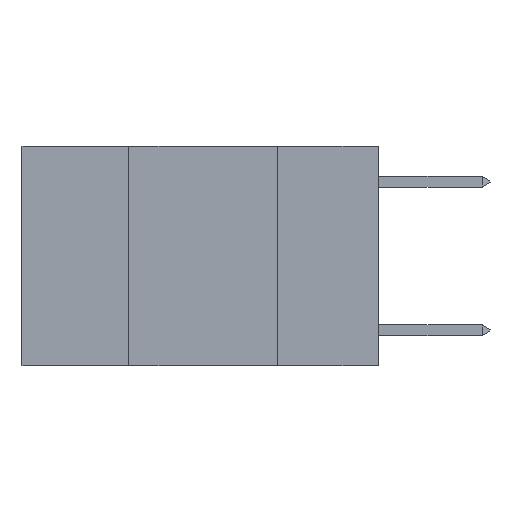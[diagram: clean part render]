
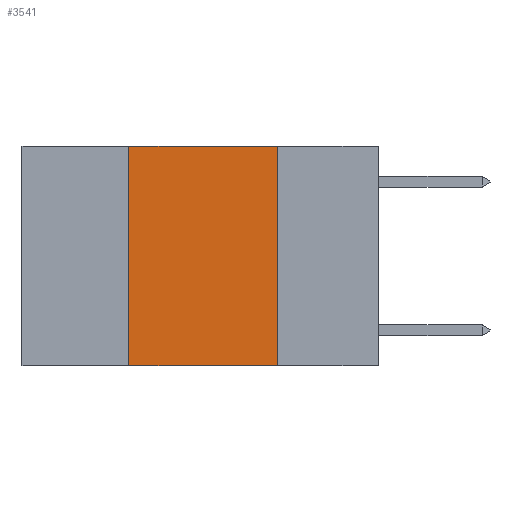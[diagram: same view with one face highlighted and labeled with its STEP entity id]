
A CAD part, left-side view. The second image highlights one B-rep face of the part: STEP entity #3541.
In plain terms, the highlighted planar face has unit normal (-1, 0, 0).
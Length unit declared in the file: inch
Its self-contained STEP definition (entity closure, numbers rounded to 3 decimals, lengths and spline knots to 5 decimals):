
#386 = ORIENTED_EDGE ( 'NONE', *, *, #5885, .F. ) ;
#1337 = VERTEX_POINT ( 'NONE', #8611 ) ;
#1564 = VECTOR ( 'NONE', #6463, 39.37008 ) ;
#2106 = VECTOR ( 'NONE', #2562, 39.37008 ) ;
#2552 = CARTESIAN_POINT ( 'NONE',  ( 0., 0.6, -0.37 ) ) ;
#2562 = DIRECTION ( 'NONE',  ( 0., -1., 0. ) ) ;
#2815 = ORIENTED_EDGE ( 'NONE', *, *, #5584, .F. ) ;
#3263 = LINE ( 'NONE', #6498, #1564 ) ;
#3357 = ORIENTED_EDGE ( 'NONE', *, *, #6048, .T. ) ;
#3540 = VERTEX_POINT ( 'NONE', #3819 ) ;
#3541 = ADVANCED_FACE ( 'NONE', ( #12477 ), #3782, .F. ) ;
#3711 = DIRECTION ( 'NONE',  ( 0., 0., -1. ) ) ;
#3741 = DIRECTION ( 'NONE',  ( 1., 0., 0. ) ) ;
#3755 = CARTESIAN_POINT ( 'NONE',  ( 0., 0.6, 0. ) ) ;
#3782 = PLANE ( 'NONE',  #4789 ) ;
#3798 = CARTESIAN_POINT ( 'NONE',  ( 0., 0.17, 0. ) ) ;
#3811 = DIRECTION ( 'NONE',  ( 0., 0., 1. ) ) ;
#3819 = CARTESIAN_POINT ( 'NONE',  ( 0., 0.42, -0.37 ) ) ;
#3984 = CARTESIAN_POINT ( 'NONE',  ( 0., 0.42, 0. ) ) ;
#4105 = LINE ( 'NONE', #2552, #2106 ) ;
#4789 = AXIS2_PLACEMENT_3D ( 'NONE', #3755, #3741, #3711 ) ;
#5584 = EDGE_CURVE ( 'NONE', #9605, #1337, #3263, .T. ) ;
#5885 = EDGE_CURVE ( 'NONE', #3540, #11742, #9350, .T. ) ;
#6048 = EDGE_CURVE ( 'NONE', #3540, #1337, #4105, .T. ) ;
#6463 = DIRECTION ( 'NONE',  ( 0., 0., -1. ) ) ;
#6498 = CARTESIAN_POINT ( 'NONE',  ( 0., 0.17, 0. ) ) ;
#7395 = VECTOR ( 'NONE', #8224, 39.37008 ) ;
#7865 = CARTESIAN_POINT ( 'NONE',  ( 0., 0.42, 0. ) ) ;
#8224 = DIRECTION ( 'NONE',  ( 0., -1., 0. ) ) ;
#8611 = CARTESIAN_POINT ( 'NONE',  ( 0., 0.17, -0.37 ) ) ;
#9176 = VECTOR ( 'NONE', #3811, 39.37008 ) ;
#9350 = LINE ( 'NONE', #3984, #9176 ) ;
#9605 = VERTEX_POINT ( 'NONE', #3798 ) ;
#10074 = EDGE_LOOP ( 'NONE', ( #2815, #12623, #386, #3357 ) ) ;
#10077 = LINE ( 'NONE', #13101, #7395 ) ;
#11742 = VERTEX_POINT ( 'NONE', #7865 ) ;
#11970 = EDGE_CURVE ( 'NONE', #11742, #9605, #10077, .T. ) ;
#12477 = FACE_OUTER_BOUND ( 'NONE', #10074, .T. ) ;
#12623 = ORIENTED_EDGE ( 'NONE', *, *, #11970, .F. ) ;
#13101 = CARTESIAN_POINT ( 'NONE',  ( 0., 0.6, 0. ) ) ;
